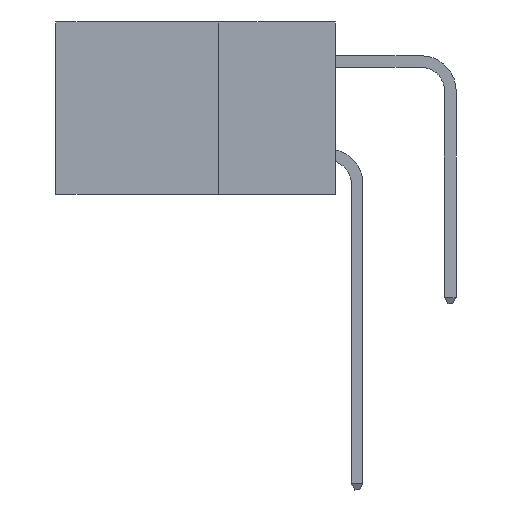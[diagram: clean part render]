
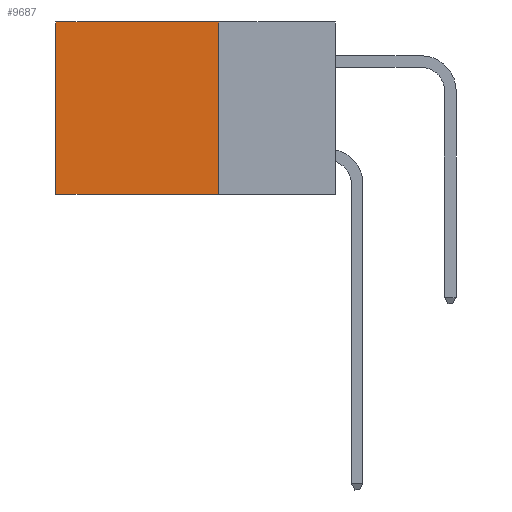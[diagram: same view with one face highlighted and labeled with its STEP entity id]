
A CAD part, left-side view. The second image highlights one B-rep face of the part: STEP entity #9687.
In plain terms, the highlighted planar face has unit normal (-1, 0, 0).
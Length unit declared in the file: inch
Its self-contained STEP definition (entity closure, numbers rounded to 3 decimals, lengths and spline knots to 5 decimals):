
#724 = DIRECTION ( 'NONE',  ( 0., 0., -1. ) ) ;
#1248 = CARTESIAN_POINT ( 'NONE',  ( 0.2875, 0.25, -0.37 ) ) ;
#1483 = LINE ( 'NONE', #6214, #1769 ) ;
#1769 = VECTOR ( 'NONE', #7060, 39.37008 ) ;
#2304 = EDGE_CURVE ( 'NONE', #2854, #8170, #12263, .T. ) ;
#2352 = ORIENTED_EDGE ( 'NONE', *, *, #10106, .T. ) ;
#2474 = CARTESIAN_POINT ( 'NONE',  ( 0.2875, 0.25, 0. ) ) ;
#2635 = CARTESIAN_POINT ( 'NONE',  ( 0.2875, 0.25, -0.37 ) ) ;
#2687 = VECTOR ( 'NONE', #3724, 39.37008 ) ;
#2854 = VERTEX_POINT ( 'NONE', #1248 ) ;
#3394 = DIRECTION ( 'NONE',  ( 0., 0., -1. ) ) ;
#3724 = DIRECTION ( 'NONE',  ( 0., 1., 0. ) ) ;
#4320 = CARTESIAN_POINT ( 'NONE',  ( 0.2875, 0.6, 0. ) ) ;
#4632 = VECTOR ( 'NONE', #3394, 39.37008 ) ;
#4724 = EDGE_CURVE ( 'NONE', #9131, #2854, #1483, .T. ) ;
#4730 = VERTEX_POINT ( 'NONE', #8158 ) ;
#4941 = EDGE_CURVE ( 'NONE', #9131, #4730, #7840, .T. ) ;
#5167 = ORIENTED_EDGE ( 'NONE', *, *, #4724, .F. ) ;
#5755 = ORIENTED_EDGE ( 'NONE', *, *, #2304, .F. ) ;
#6207 = EDGE_LOOP ( 'NONE', ( #2352, #5755, #5167, #11902 ) ) ;
#6214 = CARTESIAN_POINT ( 'NONE',  ( 0.2875, 0.25, 0. ) ) ;
#6607 = FACE_OUTER_BOUND ( 'NONE', #6207, .T. ) ;
#6907 = LINE ( 'NONE', #4320, #4632 ) ;
#7060 = DIRECTION ( 'NONE',  ( 0., 0., -1. ) ) ;
#7840 = LINE ( 'NONE', #8523, #2687 ) ;
#8158 = CARTESIAN_POINT ( 'NONE',  ( 0.2875, 0.6, 0. ) ) ;
#8170 = VERTEX_POINT ( 'NONE', #11981 ) ;
#8523 = CARTESIAN_POINT ( 'NONE',  ( 0.2875, 0.25, 0. ) ) ;
#9131 = VERTEX_POINT ( 'NONE', #2474 ) ;
#9410 = DIRECTION ( 'NONE',  ( 0., 1., 0. ) ) ;
#9501 = DIRECTION ( 'NONE',  ( 1., 0., 0. ) ) ;
#9687 = ADVANCED_FACE ( 'NONE', ( #6607 ), #12414, .F. ) ;
#9708 = VECTOR ( 'NONE', #9410, 39.37008 ) ;
#9966 = AXIS2_PLACEMENT_3D ( 'NONE', #12285, #9501, #724 ) ;
#10106 = EDGE_CURVE ( 'NONE', #4730, #8170, #6907, .T. ) ;
#11902 = ORIENTED_EDGE ( 'NONE', *, *, #4941, .T. ) ;
#11981 = CARTESIAN_POINT ( 'NONE',  ( 0.2875, 0.6, -0.37 ) ) ;
#12263 = LINE ( 'NONE', #2635, #9708 ) ;
#12285 = CARTESIAN_POINT ( 'NONE',  ( 0.2875, 0.25, 0. ) ) ;
#12414 = PLANE ( 'NONE',  #9966 ) ;
